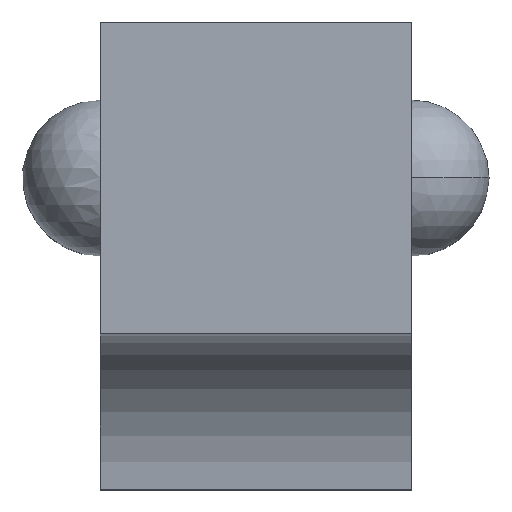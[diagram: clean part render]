
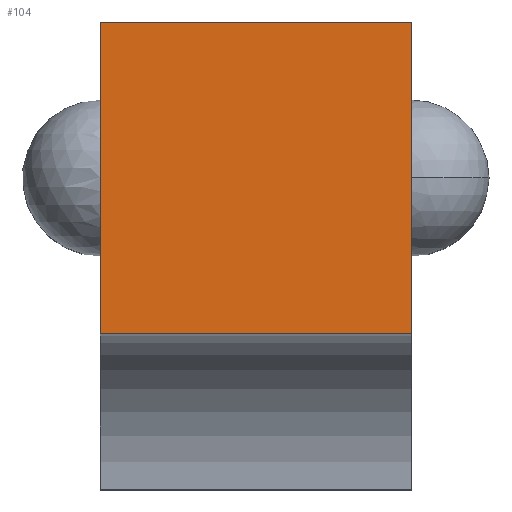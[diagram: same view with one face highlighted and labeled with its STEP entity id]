
A CAD part, top view. The second image highlights one B-rep face of the part: STEP entity #104.
In plain terms, the highlighted planar face has unit normal (0, 0, 1).
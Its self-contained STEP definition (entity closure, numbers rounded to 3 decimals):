
#11 = EDGE_CURVE ( 'NONE', #272, #275, #57, .T. ) ;
#15 = VECTOR ( 'NONE', #307, 1000. ) ;
#22 = LINE ( 'NONE', #392, #15 ) ;
#35 = EDGE_CURVE ( 'NONE', #275, #139, #22, .T. ) ;
#36 = ORIENTED_EDGE ( 'NONE', *, *, #74, .T. ) ;
#37 = VECTOR ( 'NONE', #137, 1000. ) ;
#57 = LINE ( 'NONE', #397, #37 ) ;
#64 = VERTEX_POINT ( 'NONE', #217 ) ;
#74 = EDGE_CURVE ( 'NONE', #272, #64, #376, .T. ) ;
#82 = EDGE_CURVE ( 'NONE', #64, #139, #377, .T. ) ;
#104 = ADVANCED_FACE ( 'NONE', ( #371 ), #295, .F. ) ;
#108 = CARTESIAN_POINT ( 'NONE',  ( 10., 0., 10. ) ) ;
#114 = DIRECTION ( 'NONE',  ( 0., 0., -1. ) ) ;
#133 = DIRECTION ( 'NONE',  ( 0., -1., 0. ) ) ;
#137 = DIRECTION ( 'NONE',  ( 0., -1., 0. ) ) ;
#139 = VERTEX_POINT ( 'NONE', #346 ) ;
#158 = CARTESIAN_POINT ( 'NONE',  ( 10., 20., 10. ) ) ;
#190 = CARTESIAN_POINT ( 'NONE',  ( 10., 10., 10. ) ) ;
#193 = CARTESIAN_POINT ( 'NONE',  ( 10., 20., 10. ) ) ;
#196 = VECTOR ( 'NONE', #414, 1000. ) ;
#217 = CARTESIAN_POINT ( 'NONE',  ( 0., 20., 10. ) ) ;
#234 = ORIENTED_EDGE ( 'NONE', *, *, #35, .F. ) ;
#240 = AXIS2_PLACEMENT_3D ( 'NONE', #108, #114, #288 ) ;
#255 = EDGE_LOOP ( 'NONE', ( #311, #234, #357, #36 ) ) ;
#272 = VERTEX_POINT ( 'NONE', #193 ) ;
#275 = VERTEX_POINT ( 'NONE', #190 ) ;
#283 = CARTESIAN_POINT ( 'NONE',  ( 0., 0., 10. ) ) ;
#288 = DIRECTION ( 'NONE',  ( 0., 1., 0. ) ) ;
#295 = PLANE ( 'NONE',  #240 ) ;
#307 = DIRECTION ( 'NONE',  ( -1., 0., 0. ) ) ;
#311 = ORIENTED_EDGE ( 'NONE', *, *, #82, .T. ) ;
#346 = CARTESIAN_POINT ( 'NONE',  ( 0., 10., 10. ) ) ;
#357 = ORIENTED_EDGE ( 'NONE', *, *, #11, .F. ) ;
#367 = VECTOR ( 'NONE', #133, 1000. ) ;
#371 = FACE_OUTER_BOUND ( 'NONE', #255, .T. ) ;
#376 = LINE ( 'NONE', #158, #196 ) ;
#377 = LINE ( 'NONE', #283, #367 ) ;
#392 = CARTESIAN_POINT ( 'NONE',  ( 10., 10., 10. ) ) ;
#397 = CARTESIAN_POINT ( 'NONE',  ( 10., 0., 10. ) ) ;
#414 = DIRECTION ( 'NONE',  ( -1., 0., 0. ) ) ;
